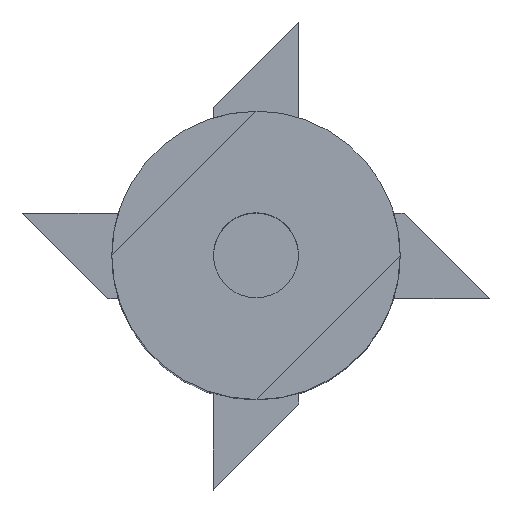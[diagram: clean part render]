
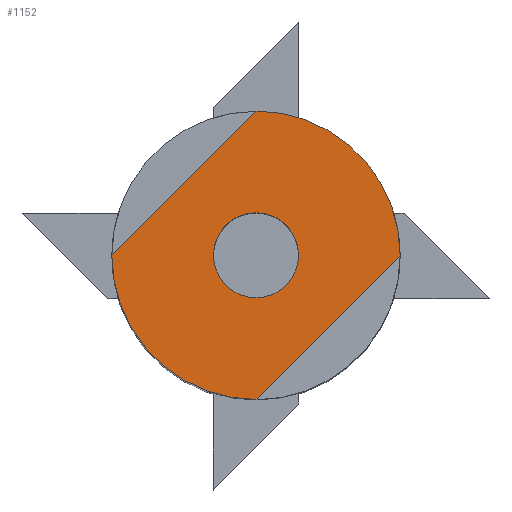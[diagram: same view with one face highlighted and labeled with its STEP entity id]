
A CAD part, top view. The second image highlights one B-rep face of the part: STEP entity #1152.
In plain terms, the highlighted planar face has unit normal (0, 0, 1).
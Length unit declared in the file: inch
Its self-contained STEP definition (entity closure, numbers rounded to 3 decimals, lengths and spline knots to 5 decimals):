
#3 = VERTEX_POINT ( 'NONE', #308 ) ;
#8 = CARTESIAN_POINT ( 'NONE',  ( 22.58257, 15.68599, 10. ) ) ;
#24 = AXIS2_PLACEMENT_3D ( 'NONE', #344, #153, #145 ) ;
#113 = ORIENTED_EDGE ( 'NONE', *, *, #826, .F. ) ;
#124 = DIRECTION ( 'NONE',  ( 1., 0., 0. ) ) ;
#127 = DIRECTION ( 'NONE',  ( 0., 0., 1. ) ) ;
#145 = DIRECTION ( 'NONE',  ( 1., 0., 0. ) ) ;
#153 = DIRECTION ( 'NONE',  ( 0., 0., 1. ) ) ;
#161 = PLANE ( 'NONE',  #24 ) ;
#182 = EDGE_LOOP ( 'NONE', ( #913, #1031, #777, #1003 ) ) ;
#194 = VECTOR ( 'NONE', #551, 39.37008 ) ;
#197 = CARTESIAN_POINT ( 'NONE',  ( 22.58257, 15.68599, 10. ) ) ;
#210 = CIRCLE ( 'NONE', #1004, 1.70412 ) ;
#308 = CARTESIAN_POINT ( 'NONE',  ( 22.58257, 17.39011, 10. ) ) ;
#336 = EDGE_LOOP ( 'NONE', ( #810, #113 ) ) ;
#344 = CARTESIAN_POINT ( 'NONE',  ( 0., 0., 10. ) ) ;
#353 = VERTEX_POINT ( 'NONE', #631 ) ;
#377 = CIRCLE ( 'NONE', #729, 0.50198 ) ;
#443 = CIRCLE ( 'NONE', #1026, 0.50198 ) ;
#480 = CARTESIAN_POINT ( 'NONE',  ( 4.30035, -4.30035, 10. ) ) ;
#550 = EDGE_CURVE ( 'NONE', #353, #794, #999, .T. ) ;
#551 = DIRECTION ( 'NONE',  ( -0.707, -0.707, 0. ) ) ;
#555 = AXIS2_PLACEMENT_3D ( 'NONE', #934, #792, #680 ) ;
#627 = EDGE_CURVE ( 'NONE', #835, #712, #443, .T. ) ;
#631 = CARTESIAN_POINT ( 'NONE',  ( 22.58257, 13.98188, 10. ) ) ;
#653 = EDGE_CURVE ( 'NONE', #794, #3, #210, .T. ) ;
#666 = CARTESIAN_POINT ( 'NONE',  ( 23.08455, 15.68599, 10. ) ) ;
#680 = DIRECTION ( 'NONE',  ( 1., 0., 0. ) ) ;
#694 = CARTESIAN_POINT ( 'NONE',  ( 20.87845, 15.68599, 10. ) ) ;
#712 = VERTEX_POINT ( 'NONE', #666 ) ;
#729 = AXIS2_PLACEMENT_3D ( 'NONE', #988, #985, #979 ) ;
#777 = ORIENTED_EDGE ( 'NONE', *, *, #653, .T. ) ;
#778 = VECTOR ( 'NONE', #997, 39.37008 ) ;
#791 = EDGE_CURVE ( 'NONE', #3, #1144, #882, .T. ) ;
#792 = DIRECTION ( 'NONE',  ( 0., 0., 1. ) ) ;
#794 = VERTEX_POINT ( 'NONE', #1164 ) ;
#810 = ORIENTED_EDGE ( 'NONE', *, *, #627, .F. ) ;
#826 = EDGE_CURVE ( 'NONE', #712, #835, #377, .T. ) ;
#835 = VERTEX_POINT ( 'NONE', #1077 ) ;
#882 = LINE ( 'NONE', #1167, #194 ) ;
#889 = CIRCLE ( 'NONE', #555, 1.70412 ) ;
#913 = ORIENTED_EDGE ( 'NONE', *, *, #928, .T. ) ;
#928 = EDGE_CURVE ( 'NONE', #1144, #353, #889, .T. ) ;
#933 = FACE_BOUND ( 'NONE', #336, .T. ) ;
#934 = CARTESIAN_POINT ( 'NONE',  ( 22.58257, 15.68599, 10. ) ) ;
#979 = DIRECTION ( 'NONE',  ( 1., 0., 0. ) ) ;
#985 = DIRECTION ( 'NONE',  ( 0., 0., 1. ) ) ;
#988 = CARTESIAN_POINT ( 'NONE',  ( 22.58257, 15.68599, 10. ) ) ;
#997 = DIRECTION ( 'NONE',  ( 0.707, 0.707, 0. ) ) ;
#999 = LINE ( 'NONE', #480, #778 ) ;
#1003 = ORIENTED_EDGE ( 'NONE', *, *, #791, .T. ) ;
#1004 = AXIS2_PLACEMENT_3D ( 'NONE', #8, #1094, #1006 ) ;
#1006 = DIRECTION ( 'NONE',  ( 1., 0., 0. ) ) ;
#1026 = AXIS2_PLACEMENT_3D ( 'NONE', #197, #127, #124 ) ;
#1031 = ORIENTED_EDGE ( 'NONE', *, *, #550, .T. ) ;
#1077 = CARTESIAN_POINT ( 'NONE',  ( 22.08059, 15.68599, 10. ) ) ;
#1094 = DIRECTION ( 'NONE',  ( 0., 0., 1. ) ) ;
#1144 = VERTEX_POINT ( 'NONE', #694 ) ;
#1150 = FACE_OUTER_BOUND ( 'NONE', #182, .T. ) ;
#1152 = ADVANCED_FACE ( 'NONE', ( #1150, #933 ), #161, .T. ) ;
#1164 = CARTESIAN_POINT ( 'NONE',  ( 24.28669, 15.68599, 10. ) ) ;
#1167 = CARTESIAN_POINT ( 'NONE',  ( 2.59623, -2.59623, 10. ) ) ;
